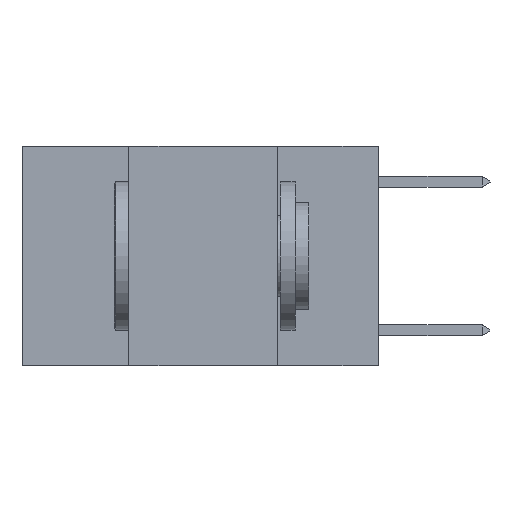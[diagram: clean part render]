
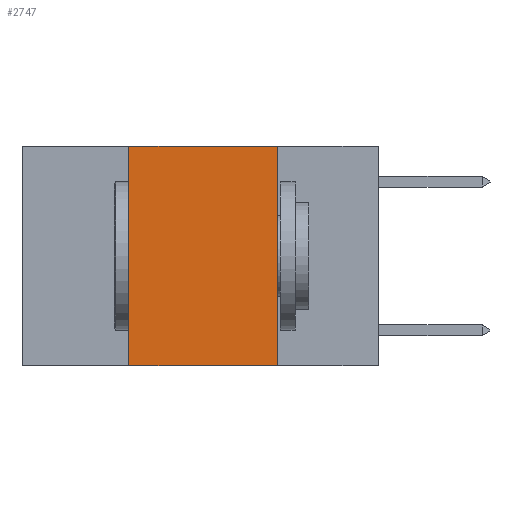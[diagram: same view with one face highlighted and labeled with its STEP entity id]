
A CAD part, left-side view. The second image highlights one B-rep face of the part: STEP entity #2747.
In plain terms, the highlighted planar face has unit normal (-1, 0, 0).
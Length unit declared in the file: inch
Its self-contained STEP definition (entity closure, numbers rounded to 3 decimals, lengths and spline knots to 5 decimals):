
#1138 = DIRECTION ( 'NONE',  ( 0., 0., -1. ) ) ;
#1306 = PLANE ( 'NONE',  #1700 ) ;
#1700 = AXIS2_PLACEMENT_3D ( 'NONE', #7363, #5082, #1138 ) ;
#1785 = VECTOR ( 'NONE', #14593, 39.37008 ) ;
#1950 = LINE ( 'NONE', #10805, #14367 ) ;
#2079 = LINE ( 'NONE', #4437, #1785 ) ;
#2511 = VECTOR ( 'NONE', #2716, 39.37008 ) ;
#2716 = DIRECTION ( 'NONE',  ( 0., 0., -1. ) ) ;
#2747 = ADVANCED_FACE ( 'NONE', ( #7530 ), #1306, .F. ) ;
#3247 = VERTEX_POINT ( 'NONE', #4196 ) ;
#3347 = EDGE_CURVE ( 'NONE', #3247, #3947, #2079, .T. ) ;
#3817 = EDGE_CURVE ( 'NONE', #3947, #13288, #14326, .T. ) ;
#3947 = VERTEX_POINT ( 'NONE', #15052 ) ;
#4164 = LINE ( 'NONE', #9035, #2511 ) ;
#4196 = CARTESIAN_POINT ( 'NONE',  ( 0., 0.42, -0.37 ) ) ;
#4198 = EDGE_CURVE ( 'NONE', #3247, #13019, #1950, .T. ) ;
#4437 = CARTESIAN_POINT ( 'NONE',  ( 0., 0.42, 0. ) ) ;
#5082 = DIRECTION ( 'NONE',  ( 1., 0., 0. ) ) ;
#5455 = VECTOR ( 'NONE', #15654, 39.37008 ) ;
#5572 = CARTESIAN_POINT ( 'NONE',  ( 0., 0.6, 0. ) ) ;
#7363 = CARTESIAN_POINT ( 'NONE',  ( 0., 0.6, 0. ) ) ;
#7530 = FACE_OUTER_BOUND ( 'NONE', #13444, .T. ) ;
#7986 = CARTESIAN_POINT ( 'NONE',  ( 0., 0.17, 0. ) ) ;
#8265 = DIRECTION ( 'NONE',  ( 0., -1., 0. ) ) ;
#9035 = CARTESIAN_POINT ( 'NONE',  ( 0., 0.17, 0. ) ) ;
#10245 = ORIENTED_EDGE ( 'NONE', *, *, #4198, .T. ) ;
#10805 = CARTESIAN_POINT ( 'NONE',  ( 0., 0.6, -0.37 ) ) ;
#11121 = CARTESIAN_POINT ( 'NONE',  ( 0., 0.17, -0.37 ) ) ;
#13019 = VERTEX_POINT ( 'NONE', #11121 ) ;
#13239 = ORIENTED_EDGE ( 'NONE', *, *, #3347, .F. ) ;
#13288 = VERTEX_POINT ( 'NONE', #7986 ) ;
#13444 = EDGE_LOOP ( 'NONE', ( #15299, #14448, #13239, #10245 ) ) ;
#14326 = LINE ( 'NONE', #5572, #5455 ) ;
#14367 = VECTOR ( 'NONE', #8265, 39.37008 ) ;
#14448 = ORIENTED_EDGE ( 'NONE', *, *, #3817, .F. ) ;
#14593 = DIRECTION ( 'NONE',  ( 0., 0., 1. ) ) ;
#15052 = CARTESIAN_POINT ( 'NONE',  ( 0., 0.42, 0. ) ) ;
#15299 = ORIENTED_EDGE ( 'NONE', *, *, #16222, .F. ) ;
#15654 = DIRECTION ( 'NONE',  ( 0., -1., 0. ) ) ;
#16222 = EDGE_CURVE ( 'NONE', #13288, #13019, #4164, .T. ) ;
